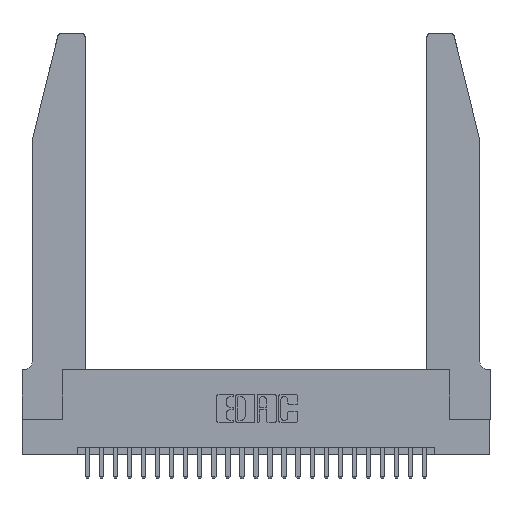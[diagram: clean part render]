
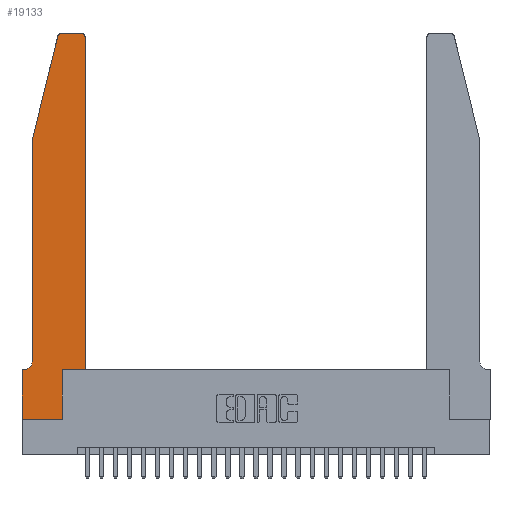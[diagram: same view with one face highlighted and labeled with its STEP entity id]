
A CAD part, top view. The second image highlights one B-rep face of the part: STEP entity #19133.
In plain terms, the highlighted planar face has unit normal (0, 0, 1).
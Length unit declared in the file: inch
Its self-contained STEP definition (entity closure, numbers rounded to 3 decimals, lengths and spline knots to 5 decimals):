
#182 = DIRECTION ( 'NONE',  ( -1., 0., 0. ) ) ;
#689 = CARTESIAN_POINT ( 'NONE',  ( 0.0055, 0.35, 0.37 ) ) ;
#731 = LINE ( 'NONE', #24710, #25246 ) ;
#866 = EDGE_CURVE ( 'NONE', #16181, #23334, #4826, .T. ) ;
#1850 = VECTOR ( 'NONE', #18456, 39.37008 ) ;
#1962 = ORIENTED_EDGE ( 'NONE', *, *, #8799, .T. ) ;
#2790 = LINE ( 'NONE', #18924, #16057 ) ;
#2905 = ORIENTED_EDGE ( 'NONE', *, *, #9390, .T. ) ;
#3014 = ORIENTED_EDGE ( 'NONE', *, *, #12455, .T. ) ;
#3090 = CARTESIAN_POINT ( 'NONE',  ( 0.0755, 0.35, 0.37 ) ) ;
#3279 = DIRECTION ( 'NONE',  ( 1., 0., 0. ) ) ;
#3446 = DIRECTION ( 'NONE',  ( 1., 0., 0. ) ) ;
#3540 = CARTESIAN_POINT ( 'NONE',  ( 0.4505, 0.35, 0.37 ) ) ;
#3600 = CARTESIAN_POINT ( 'NONE',  ( 0.2865, 0.35, 0.37 ) ) ;
#4202 = DIRECTION ( 'NONE',  ( 1., 0., 0. ) ) ;
#4250 = CARTESIAN_POINT ( 'NONE',  ( 0.4505, 2.72, 0.37 ) ) ;
#4396 = VECTOR ( 'NONE', #9524, 39.37008 ) ;
#4597 = EDGE_CURVE ( 'NONE', #21776, #16181, #731, .T. ) ;
#4826 = CIRCLE ( 'NONE', #13271, 0.03 ) ;
#5019 = DIRECTION ( 'NONE',  ( 0., 0., 1. ) ) ;
#5146 = EDGE_CURVE ( 'NONE', #23334, #5989, #23600, .T. ) ;
#5194 = DIRECTION ( 'NONE',  ( 0., 1., 0. ) ) ;
#5942 = DIRECTION ( 'NONE',  ( 0., 0., 1. ) ) ;
#5954 = CARTESIAN_POINT ( 'NONE',  ( 0., 0.35, 0.37 ) ) ;
#5989 = VERTEX_POINT ( 'NONE', #9022 ) ;
#7416 = FACE_OUTER_BOUND ( 'NONE', #12032, .T. ) ;
#7484 = EDGE_CURVE ( 'NONE', #13444, #9056, #18314, .T. ) ;
#7501 = ORIENTED_EDGE ( 'NONE', *, *, #866, .T. ) ;
#7682 = VERTEX_POINT ( 'NONE', #17050 ) ;
#7884 = CARTESIAN_POINT ( 'NONE',  ( 0.0755, 0.42, 0.37 ) ) ;
#8559 = CARTESIAN_POINT ( 'NONE',  ( 0.4505, 0.35, 0.37 ) ) ;
#8799 = EDGE_CURVE ( 'NONE', #9056, #16800, #14717, .T. ) ;
#9022 = CARTESIAN_POINT ( 'NONE',  ( 0.0755, 2., 0.37 ) ) ;
#9056 = VERTEX_POINT ( 'NONE', #19036 ) ;
#9390 = EDGE_CURVE ( 'NONE', #25797, #9622, #23038, .T. ) ;
#9524 = DIRECTION ( 'NONE',  ( -1., 0., 0. ) ) ;
#9622 = VERTEX_POINT ( 'NONE', #689 ) ;
#10204 = EDGE_CURVE ( 'NONE', #16392, #21776, #17051, .T. ) ;
#10277 = DIRECTION ( 'NONE',  ( -1., 0., 0. ) ) ;
#10344 = CARTESIAN_POINT ( 'NONE',  ( 0.25487, 2.72718, 0.37 ) ) ;
#10726 = DIRECTION ( 'NONE',  ( 0., -1., 0. ) ) ;
#10867 = DIRECTION ( 'NONE',  ( 0., 0., -1. ) ) ;
#11866 = ORIENTED_EDGE ( 'NONE', *, *, #4597, .T. ) ;
#11934 = DIRECTION ( 'NONE',  ( 1., 0., 0. ) ) ;
#12032 = EDGE_LOOP ( 'NONE', ( #11866, #7501, #24424, #16552, #2905, #18336, #23305, #15892, #1962, #3014, #13184, #18395 ) ) ;
#12455 = EDGE_CURVE ( 'NONE', #16800, #7682, #17267, .T. ) ;
#12539 = VECTOR ( 'NONE', #4202, 39.37008 ) ;
#12829 = LINE ( 'NONE', #3090, #4396 ) ;
#13041 = CARTESIAN_POINT ( 'NONE',  ( 0.4205, 2.75, 0.37 ) ) ;
#13184 = ORIENTED_EDGE ( 'NONE', *, *, #15067, .T. ) ;
#13220 = AXIS2_PLACEMENT_3D ( 'NONE', #26259, #20104, #19840 ) ;
#13271 = AXIS2_PLACEMENT_3D ( 'NONE', #15440, #5019, #3279 ) ;
#13444 = VERTEX_POINT ( 'NONE', #16794 ) ;
#13646 = DIRECTION ( 'NONE',  ( 0., 1., 0. ) ) ;
#14122 = CARTESIAN_POINT ( 'NONE',  ( 0., 0.35, 0.37 ) ) ;
#14222 = VECTOR ( 'NONE', #13646, 39.37008 ) ;
#14717 = LINE ( 'NONE', #17835, #20859 ) ;
#15067 = EDGE_CURVE ( 'NONE', #7682, #16392, #23904, .T. ) ;
#15440 = CARTESIAN_POINT ( 'NONE',  ( 0.284, 2.72, 0.37 ) ) ;
#15892 = ORIENTED_EDGE ( 'NONE', *, *, #7484, .T. ) ;
#16057 = VECTOR ( 'NONE', #10726, 39.37008 ) ;
#16181 = VERTEX_POINT ( 'NONE', #18087 ) ;
#16296 = VECTOR ( 'NONE', #3446, 39.37008 ) ;
#16392 = VERTEX_POINT ( 'NONE', #4250 ) ;
#16552 = ORIENTED_EDGE ( 'NONE', *, *, #23881, .T. ) ;
#16794 = CARTESIAN_POINT ( 'NONE',  ( 0., 0., 0.37 ) ) ;
#16800 = VERTEX_POINT ( 'NONE', #3600 ) ;
#16872 = CARTESIAN_POINT ( 'NONE',  ( 0., 0., 0.37 ) ) ;
#17050 = CARTESIAN_POINT ( 'NONE',  ( 0.4505, 0.35, 0.37 ) ) ;
#17051 = CIRCLE ( 'NONE', #13220, 0.03 ) ;
#17267 = LINE ( 'NONE', #3540, #16296 ) ;
#17835 = CARTESIAN_POINT ( 'NONE',  ( 0.2865, 0.35, 0.37 ) ) ;
#18087 = CARTESIAN_POINT ( 'NONE',  ( 0.284, 2.75, 0.37 ) ) ;
#18314 = LINE ( 'NONE', #16872, #12539 ) ;
#18336 = ORIENTED_EDGE ( 'NONE', *, *, #21366, .T. ) ;
#18358 = LINE ( 'NONE', #22800, #1850 ) ;
#18395 = ORIENTED_EDGE ( 'NONE', *, *, #10204, .T. ) ;
#18456 = DIRECTION ( 'NONE',  ( 0., -1., 0. ) ) ;
#18924 = CARTESIAN_POINT ( 'NONE',  ( 0., 0., 0.37 ) ) ;
#19036 = CARTESIAN_POINT ( 'NONE',  ( 0.2865, 0., 0.37 ) ) ;
#19133 = ADVANCED_FACE ( 'NONE', ( #7416 ), #22573, .T. ) ;
#19840 = DIRECTION ( 'NONE',  ( 1., 0., 0. ) ) ;
#20104 = DIRECTION ( 'NONE',  ( 0., 0., 1. ) ) ;
#20259 = CARTESIAN_POINT ( 'NONE',  ( 0.0755, 2., 0.37 ) ) ;
#20859 = VECTOR ( 'NONE', #5194, 39.37008 ) ;
#21080 = EDGE_CURVE ( 'NONE', #24540, #13444, #2790, .T. ) ;
#21366 = EDGE_CURVE ( 'NONE', #9622, #24540, #12829, .T. ) ;
#21776 = VERTEX_POINT ( 'NONE', #13041 ) ;
#22041 = AXIS2_PLACEMENT_3D ( 'NONE', #14122, #5942, #11934 ) ;
#22331 = DIRECTION ( 'NONE',  ( -0.239, -0.971, 0. ) ) ;
#22573 = PLANE ( 'NONE',  #22041 ) ;
#22800 = CARTESIAN_POINT ( 'NONE',  ( 0.0755, 2., 0.37 ) ) ;
#22956 = CARTESIAN_POINT ( 'NONE',  ( 0.0055, 0.42, 0.37 ) ) ;
#23038 = CIRCLE ( 'NONE', #23437, 0.07 ) ;
#23305 = ORIENTED_EDGE ( 'NONE', *, *, #21080, .T. ) ;
#23334 = VERTEX_POINT ( 'NONE', #10344 ) ;
#23437 = AXIS2_PLACEMENT_3D ( 'NONE', #22956, #10867, #182 ) ;
#23600 = LINE ( 'NONE', #20259, #24871 ) ;
#23881 = EDGE_CURVE ( 'NONE', #5989, #25797, #18358, .T. ) ;
#23904 = LINE ( 'NONE', #8559, #14222 ) ;
#24424 = ORIENTED_EDGE ( 'NONE', *, *, #5146, .T. ) ;
#24540 = VERTEX_POINT ( 'NONE', #5954 ) ;
#24710 = CARTESIAN_POINT ( 'NONE',  ( 0.2605, 2.75, 0.37 ) ) ;
#24871 = VECTOR ( 'NONE', #22331, 39.37008 ) ;
#25246 = VECTOR ( 'NONE', #10277, 39.37008 ) ;
#25797 = VERTEX_POINT ( 'NONE', #7884 ) ;
#26259 = CARTESIAN_POINT ( 'NONE',  ( 0.4205, 2.72, 0.37 ) ) ;
